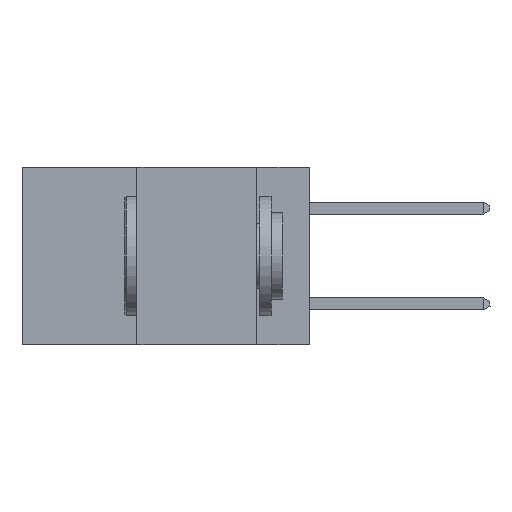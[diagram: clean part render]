
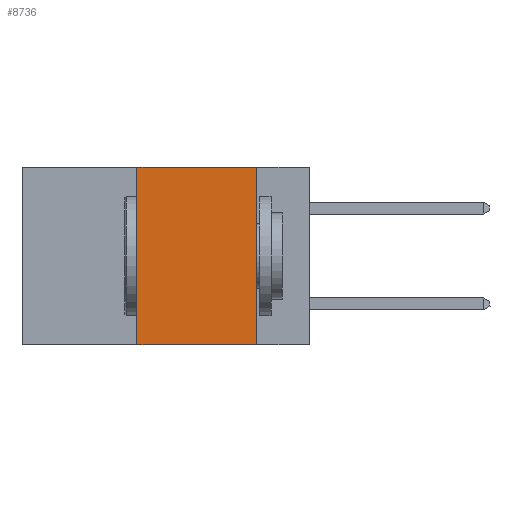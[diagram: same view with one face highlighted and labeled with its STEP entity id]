
A CAD part, left-side view. The second image highlights one B-rep face of the part: STEP entity #8736.
In plain terms, the highlighted planar face has unit normal (-1, 0, 0).
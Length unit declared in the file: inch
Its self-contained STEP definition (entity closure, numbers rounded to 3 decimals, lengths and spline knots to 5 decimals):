
#155 = CARTESIAN_POINT ( 'NONE',  ( 0., 0.6, 0. ) ) ;
#783 = VERTEX_POINT ( 'NONE', #17940 ) ;
#1305 = EDGE_CURVE ( 'NONE', #783, #14070, #12810, .T. ) ;
#1812 = DIRECTION ( 'NONE',  ( 0., -1., 0. ) ) ;
#1924 = CARTESIAN_POINT ( 'NONE',  ( 0., 0.6, 0. ) ) ;
#2284 = VERTEX_POINT ( 'NONE', #6964 ) ;
#3037 = ORIENTED_EDGE ( 'NONE', *, *, #19350, .T. ) ;
#4451 = CARTESIAN_POINT ( 'NONE',  ( 0., 0.36, 0. ) ) ;
#5068 = LINE ( 'NONE', #9779, #14114 ) ;
#5155 = DIRECTION ( 'NONE',  ( 0., 0., -1. ) ) ;
#6069 = DIRECTION ( 'NONE',  ( 0., 0., 1. ) ) ;
#6459 = EDGE_CURVE ( 'NONE', #2284, #19137, #9746, .T. ) ;
#6964 = CARTESIAN_POINT ( 'NONE',  ( 0., 0.36, -0.37 ) ) ;
#7722 = DIRECTION ( 'NONE',  ( 0., 0., -1. ) ) ;
#7748 = ORIENTED_EDGE ( 'NONE', *, *, #1305, .F. ) ;
#7773 = FACE_OUTER_BOUND ( 'NONE', #11265, .T. ) ;
#8189 = ORIENTED_EDGE ( 'NONE', *, *, #9954, .F. ) ;
#8455 = VECTOR ( 'NONE', #7722, 39.37008 ) ;
#8736 = ADVANCED_FACE ( 'NONE', ( #7773 ), #13132, .F. ) ;
#9746 = LINE ( 'NONE', #4451, #17409 ) ;
#9779 = CARTESIAN_POINT ( 'NONE',  ( 0., 0.6, -0.37 ) ) ;
#9954 = EDGE_CURVE ( 'NONE', #19137, #783, #16308, .T. ) ;
#10816 = CARTESIAN_POINT ( 'NONE',  ( 0., 0.11, 0. ) ) ;
#11265 = EDGE_LOOP ( 'NONE', ( #7748, #8189, #16927, #3037 ) ) ;
#11447 = VECTOR ( 'NONE', #1812, 39.37008 ) ;
#11872 = AXIS2_PLACEMENT_3D ( 'NONE', #1924, #14781, #5155 ) ;
#12810 = LINE ( 'NONE', #10816, #8455 ) ;
#13132 = PLANE ( 'NONE',  #11872 ) ;
#14070 = VERTEX_POINT ( 'NONE', #19809 ) ;
#14114 = VECTOR ( 'NONE', #17905, 39.37008 ) ;
#14253 = CARTESIAN_POINT ( 'NONE',  ( 0., 0.36, 0. ) ) ;
#14781 = DIRECTION ( 'NONE',  ( 1., 0., 0. ) ) ;
#16308 = LINE ( 'NONE', #155, #11447 ) ;
#16927 = ORIENTED_EDGE ( 'NONE', *, *, #6459, .F. ) ;
#17409 = VECTOR ( 'NONE', #6069, 39.37008 ) ;
#17905 = DIRECTION ( 'NONE',  ( 0., -1., 0. ) ) ;
#17940 = CARTESIAN_POINT ( 'NONE',  ( 0., 0.11, 0. ) ) ;
#19137 = VERTEX_POINT ( 'NONE', #14253 ) ;
#19350 = EDGE_CURVE ( 'NONE', #2284, #14070, #5068, .T. ) ;
#19809 = CARTESIAN_POINT ( 'NONE',  ( 0., 0.11, -0.37 ) ) ;
